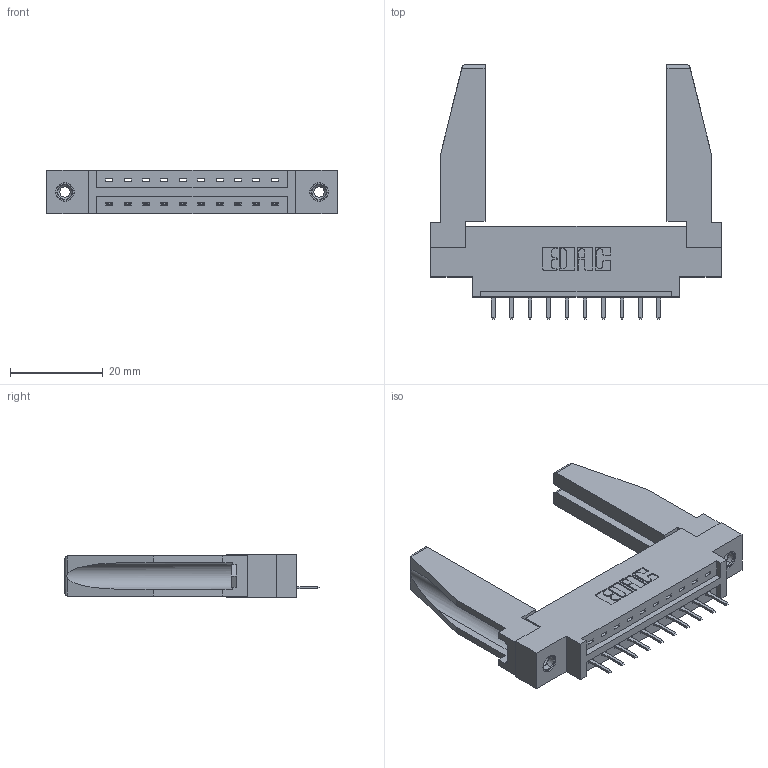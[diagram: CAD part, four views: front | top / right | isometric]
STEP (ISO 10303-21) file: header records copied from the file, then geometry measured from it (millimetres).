
FILE_DESCRIPTION (( 'STEP AP203' ), '1' );
FILE_NAME ('387-010-520-678.STEP', '2019-10-02T11:03:29', ( '' ), ( '' ), 'SwSTEP 2.0', 'SolidWorks 2016', '' );
FILE_SCHEMA (( 'CONFIG_CONTROL_DESIGN' ));
Length unit declared in the file: inch
Products named in the file (5): 307-220-078; 345-292-001_345-293-120; 337 Part_0.170 Offset - 0.156 Dia-TI; 387-010-520-678; 345-250-001_345-250-001-102
Assembly tree (15 placements, depth 2):
  387-010-520-678
    337 Part_0.170 Offset - 0.156 Dia-TI
    345-292-001_345-293-120  x10
    345-250-001_345-250-001-102  x2
    307-220-078  x2
Bounding box: 62.64 x 54.82 x 9.4 mm (x, y, z)
Volume: 9956.6 mm3; surface area: 9814.3 mm2
Topology: 15 solids, 15 shells, 908 faces, 2613 edges, 1706 vertices
Faces by surface type: plane 638, cylinder 254, cone 12, torus 4
Entity records: 14258 total; most frequent: CARTESIAN_POINT 2486, ORIENTED_EDGE 2376, DIRECTION 2156, EDGE_CURVE 1188, VECTOR 1018, LINE 1018, VERTEX_POINT 784, AXIS2_PLACEMENT_3D 569
